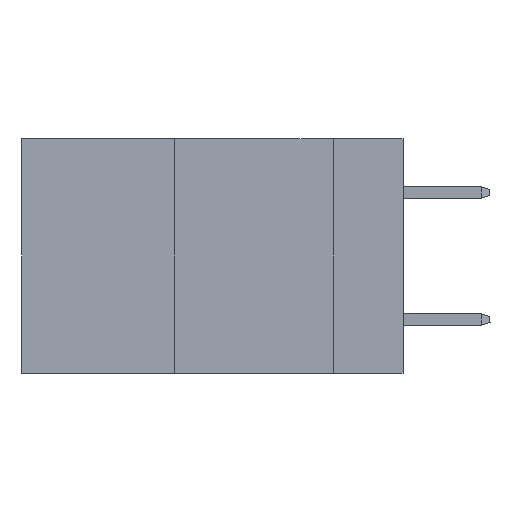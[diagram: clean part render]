
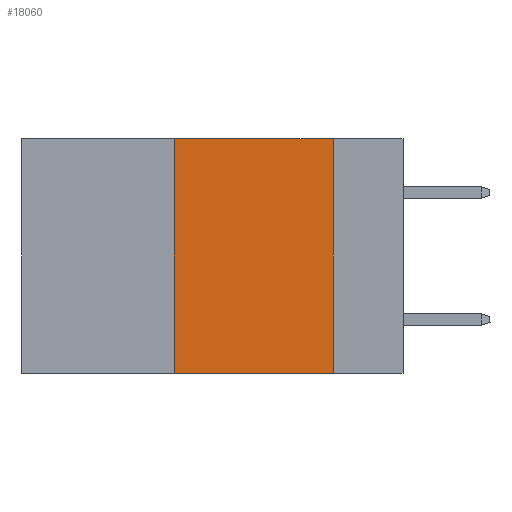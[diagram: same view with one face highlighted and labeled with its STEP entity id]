
A CAD part, left-side view. The second image highlights one B-rep face of the part: STEP entity #18060.
In plain terms, the highlighted planar face has unit normal (-1, 0, 0).
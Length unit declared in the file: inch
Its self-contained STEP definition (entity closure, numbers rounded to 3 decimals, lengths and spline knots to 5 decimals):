
#1090 = LINE ( 'NONE', #20147, #6686 ) ;
#1182 = VECTOR ( 'NONE', #10358, 39.37008 ) ;
#1519 = EDGE_CURVE ( 'NONE', #9536, #20653, #15722, .T. ) ;
#2591 = DIRECTION ( 'NONE',  ( 0., 0., 1. ) ) ;
#4621 = EDGE_CURVE ( 'NONE', #21021, #22969, #8617, .T. ) ;
#4765 = DIRECTION ( 'NONE',  ( 0., 0., -1. ) ) ;
#6686 = VECTOR ( 'NONE', #10750, 39.37008 ) ;
#6886 = DIRECTION ( 'NONE',  ( 1., 0., 0. ) ) ;
#7389 = EDGE_CURVE ( 'NONE', #20653, #21021, #1090, .T. ) ;
#8617 = LINE ( 'NONE', #19865, #1182 ) ;
#9536 = VERTEX_POINT ( 'NONE', #23006 ) ;
#10061 = EDGE_LOOP ( 'NONE', ( #14628, #21809, #14801, #16183 ) ) ;
#10358 = DIRECTION ( 'NONE',  ( 0., 0., -1. ) ) ;
#10750 = DIRECTION ( 'NONE',  ( 0., -1., 0. ) ) ;
#11725 = DIRECTION ( 'NONE',  ( 0., -1., 0. ) ) ;
#11835 = CARTESIAN_POINT ( 'NONE',  ( 0., 0.11, -0.37 ) ) ;
#12007 = VECTOR ( 'NONE', #11725, 39.37008 ) ;
#13110 = LINE ( 'NONE', #24617, #12007 ) ;
#14628 = ORIENTED_EDGE ( 'NONE', *, *, #4621, .F. ) ;
#14801 = ORIENTED_EDGE ( 'NONE', *, *, #1519, .F. ) ;
#15722 = LINE ( 'NONE', #23367, #20409 ) ;
#16183 = ORIENTED_EDGE ( 'NONE', *, *, #24449, .T. ) ;
#17767 = FACE_OUTER_BOUND ( 'NONE', #10061, .T. ) ;
#18060 = ADVANCED_FACE ( 'NONE', ( #17767 ), #24257, .F. ) ;
#19865 = CARTESIAN_POINT ( 'NONE',  ( 0., 0.11, 0. ) ) ;
#19886 = CARTESIAN_POINT ( 'NONE',  ( 0., 0.6, 0. ) ) ;
#20147 = CARTESIAN_POINT ( 'NONE',  ( 0., 0.6, 0. ) ) ;
#20409 = VECTOR ( 'NONE', #2591, 39.37008 ) ;
#20653 = VERTEX_POINT ( 'NONE', #21140 ) ;
#21021 = VERTEX_POINT ( 'NONE', #23505 ) ;
#21140 = CARTESIAN_POINT ( 'NONE',  ( 0., 0.36, 0. ) ) ;
#21809 = ORIENTED_EDGE ( 'NONE', *, *, #7389, .F. ) ;
#22969 = VERTEX_POINT ( 'NONE', #11835 ) ;
#23006 = CARTESIAN_POINT ( 'NONE',  ( 0., 0.36, -0.37 ) ) ;
#23367 = CARTESIAN_POINT ( 'NONE',  ( 0., 0.36, 0. ) ) ;
#23505 = CARTESIAN_POINT ( 'NONE',  ( 0., 0.11, 0. ) ) ;
#23527 = AXIS2_PLACEMENT_3D ( 'NONE', #19886, #6886, #4765 ) ;
#24257 = PLANE ( 'NONE',  #23527 ) ;
#24449 = EDGE_CURVE ( 'NONE', #9536, #22969, #13110, .T. ) ;
#24617 = CARTESIAN_POINT ( 'NONE',  ( 0., 0.6, -0.37 ) ) ;
